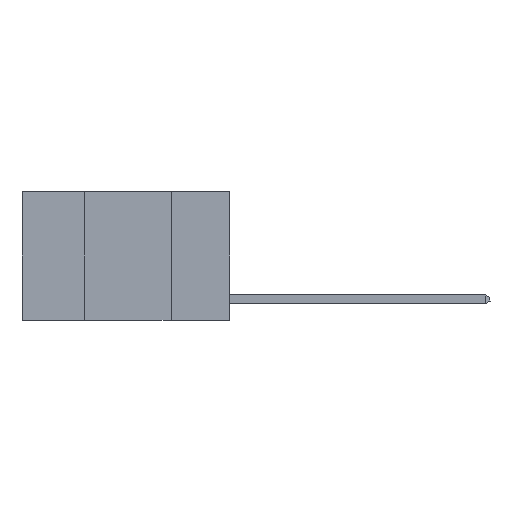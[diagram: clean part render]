
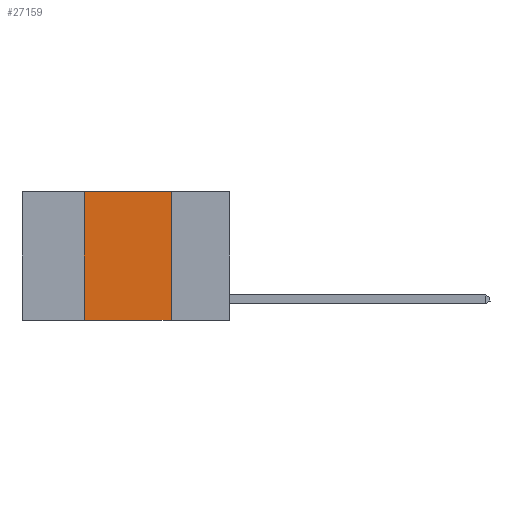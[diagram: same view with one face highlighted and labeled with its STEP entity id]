
A CAD part, left-side view. The second image highlights one B-rep face of the part: STEP entity #27159.
In plain terms, the highlighted planar face has unit normal (-1, 0, 0).
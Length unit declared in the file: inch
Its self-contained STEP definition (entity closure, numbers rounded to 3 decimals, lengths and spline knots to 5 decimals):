
#1449 = EDGE_CURVE ( 'NONE', #5303, #27294, #13495, .T. ) ;
#1912 = ORIENTED_EDGE ( 'NONE', *, *, #20928, .T. ) ;
#2630 = DIRECTION ( 'NONE',  ( 0., 0., -1. ) ) ;
#5089 = CARTESIAN_POINT ( 'NONE',  ( 0., 0.42, -0.37 ) ) ;
#5303 = VERTEX_POINT ( 'NONE', #8365 ) ;
#6254 = LINE ( 'NONE', #12278, #23729 ) ;
#6851 = ORIENTED_EDGE ( 'NONE', *, *, #14385, .F. ) ;
#8365 = CARTESIAN_POINT ( 'NONE',  ( 0., 0.42, 0. ) ) ;
#9862 = VECTOR ( 'NONE', #30671, 39.37008 ) ;
#10611 = DIRECTION ( 'NONE',  ( 0., -1., 0. ) ) ;
#12278 = CARTESIAN_POINT ( 'NONE',  ( 0., 0.42, 0. ) ) ;
#12755 = CARTESIAN_POINT ( 'NONE',  ( 0., 0.17, 0. ) ) ;
#13495 = LINE ( 'NONE', #27153, #16825 ) ;
#13518 = FACE_OUTER_BOUND ( 'NONE', #19003, .T. ) ;
#13679 = AXIS2_PLACEMENT_3D ( 'NONE', #14640, #17028, #2630 ) ;
#14385 = EDGE_CURVE ( 'NONE', #27294, #23223, #16212, .T. ) ;
#14506 = VERTEX_POINT ( 'NONE', #5089 ) ;
#14640 = CARTESIAN_POINT ( 'NONE',  ( 0., 0.6, 0. ) ) ;
#14721 = CARTESIAN_POINT ( 'NONE',  ( 0., 0.6, -0.37 ) ) ;
#16212 = LINE ( 'NONE', #16603, #9862 ) ;
#16603 = CARTESIAN_POINT ( 'NONE',  ( 0., 0.17, 0. ) ) ;
#16671 = CARTESIAN_POINT ( 'NONE',  ( 0., 0.17, -0.37 ) ) ;
#16825 = VECTOR ( 'NONE', #10611, 39.37008 ) ;
#17028 = DIRECTION ( 'NONE',  ( 1., 0., 0. ) ) ;
#17111 = DIRECTION ( 'NONE',  ( 0., -1., 0. ) ) ;
#17289 = VECTOR ( 'NONE', #17111, 39.37008 ) ;
#19003 = EDGE_LOOP ( 'NONE', ( #6851, #25792, #20292, #1912 ) ) ;
#20292 = ORIENTED_EDGE ( 'NONE', *, *, #28952, .F. ) ;
#20928 = EDGE_CURVE ( 'NONE', #14506, #23223, #23531, .T. ) ;
#23223 = VERTEX_POINT ( 'NONE', #16671 ) ;
#23531 = LINE ( 'NONE', #14721, #17289 ) ;
#23729 = VECTOR ( 'NONE', #26526, 39.37008 ) ;
#25792 = ORIENTED_EDGE ( 'NONE', *, *, #1449, .F. ) ;
#26526 = DIRECTION ( 'NONE',  ( 0., 0., 1. ) ) ;
#27153 = CARTESIAN_POINT ( 'NONE',  ( 0., 0.6, 0. ) ) ;
#27159 = ADVANCED_FACE ( 'NONE', ( #13518 ), #28753, .F. ) ;
#27294 = VERTEX_POINT ( 'NONE', #12755 ) ;
#28753 = PLANE ( 'NONE',  #13679 ) ;
#28952 = EDGE_CURVE ( 'NONE', #14506, #5303, #6254, .T. ) ;
#30671 = DIRECTION ( 'NONE',  ( 0., 0., -1. ) ) ;
